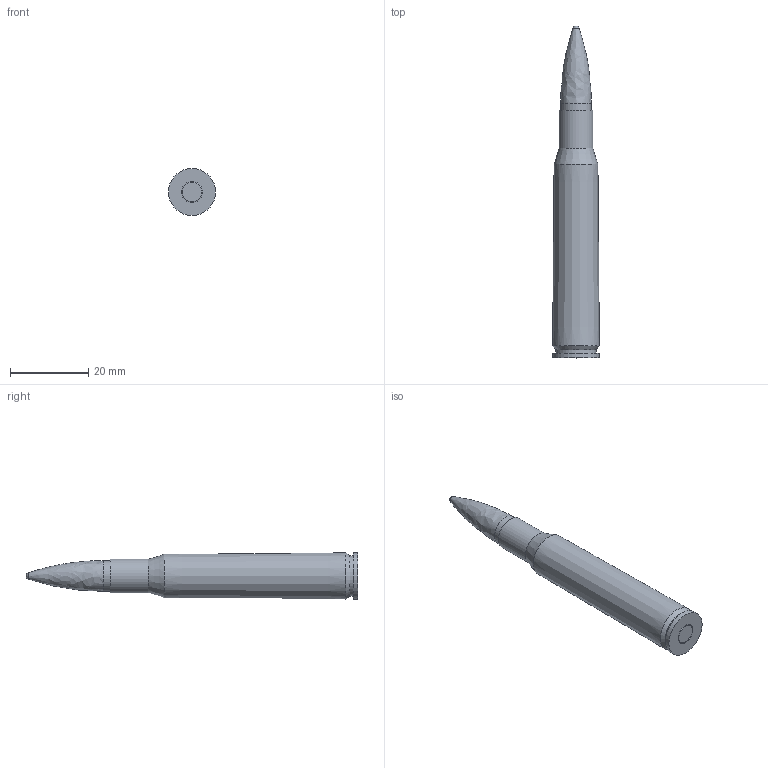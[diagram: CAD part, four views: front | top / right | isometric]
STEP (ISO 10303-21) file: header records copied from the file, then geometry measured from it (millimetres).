
FILE_DESCRIPTION((''),'2;1');
FILE_NAME('30-06 Springfield.stp','2012-11-15T13:02:53',('agarrett'),(''),'Autodesk Inventor 2012','Autodesk Inventor 2012','');
FILE_SCHEMA(('AUTOMOTIVE_DESIGN { 1 0 10303 214 1 1 1 1 }'));
Length unit declared in the file: inch
Products named in the file (6): iLogic Cartridge; iLogicCartridge; PRIMER; iLogic Bullet Chooser; iLogic Bullet; iLogic RN Bullet
Assembly tree (5 placements, depth 3):
  iLogic Cartridge
    iLogicCartridge
    PRIMER
    iLogic Bullet Chooser
      iLogic Bullet
      iLogic RN Bullet
Bounding box: 12.01 x 84.83 x 12.01 mm (x, y, z)
Volume: 7462.6 mm3; surface area: 3465.9 mm2
Topology: 3 solids, 3 shells, 24 faces, 35 edges, 21 vertices
Faces by surface type: plane 9, cylinder 8, cone 3, torus 2, sphere 1, bspline 1
Full cylindrical faces by diameter (mm): 1.778 x1, 5.08 x1, 5.334 x2, 7.849 x1, 8.628 x1, 10.389 x1, 12.014 x1
Entity records: 666 total; most frequent: DIRECTION 110, CARTESIAN_POINT 103, AXIS2_PLACEMENT_3D 55, ORIENTED_EDGE 42, EDGE_LOOP 42, FACE_OUTER_BOUND 24, ADVANCED_FACE 24, VERTEX_POINT 21
